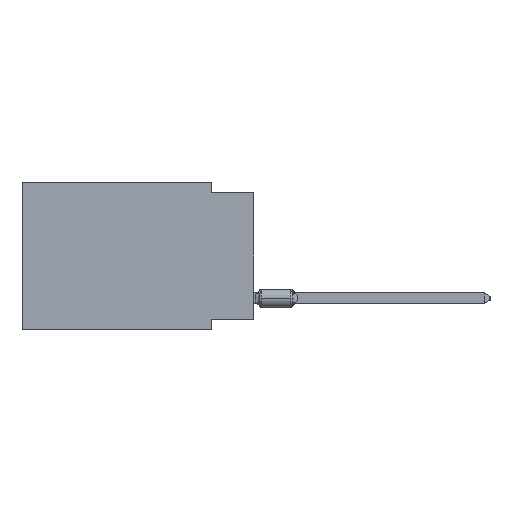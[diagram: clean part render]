
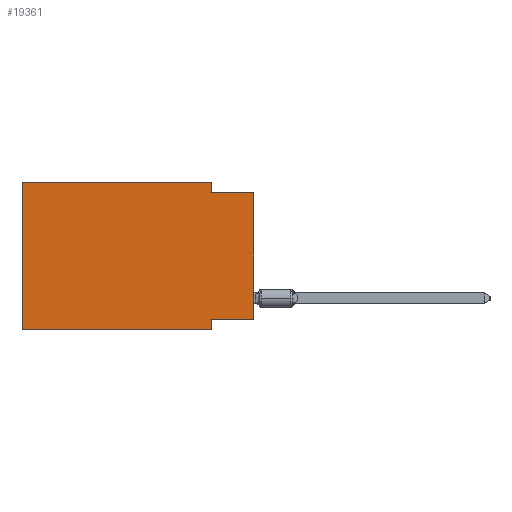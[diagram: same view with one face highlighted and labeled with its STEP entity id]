
A CAD part, left-side view. The second image highlights one B-rep face of the part: STEP entity #19361.
In plain terms, the highlighted planar face has unit normal (-1, 0, 0).
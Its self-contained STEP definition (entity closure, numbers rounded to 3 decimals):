
#1639 = ORIENTED_EDGE ( 'NONE', *, *, #43467, .F. ) ;
#3488 = DIRECTION ( 'NONE',  ( 0., 0., 1. ) ) ;
#3862 = ORIENTED_EDGE ( 'NONE', *, *, #51844, .T. ) ;
#6114 = DIRECTION ( 'NONE',  ( 0., -1., 0. ) ) ;
#6703 = EDGE_CURVE ( 'NONE', #42554, #51807, #19108, .T. ) ;
#8383 = EDGE_CURVE ( 'NONE', #15326, #42554, #37572, .T. ) ;
#8854 = AXIS2_PLACEMENT_3D ( 'NONE', #10410, #52341, #43872 ) ;
#9474 = EDGE_LOOP ( 'NONE', ( #3862, #1639, #18392, #10785, #9512, #40778, #19941, #19553 ) ) ;
#9512 = ORIENTED_EDGE ( 'NONE', *, *, #19896, .F. ) ;
#10410 = CARTESIAN_POINT ( 'NONE',  ( 0., 13.97, 0. ) ) ;
#10785 = ORIENTED_EDGE ( 'NONE', *, *, #8383, .F. ) ;
#12265 = VERTEX_POINT ( 'NONE', #48826 ) ;
#13125 = VERTEX_POINT ( 'NONE', #30211 ) ;
#13335 = CARTESIAN_POINT ( 'NONE',  ( 0., 2.54, -8.255 ) ) ;
#13735 = LINE ( 'NONE', #21696, #19118 ) ;
#15326 = VERTEX_POINT ( 'NONE', #28820 ) ;
#15983 = CARTESIAN_POINT ( 'NONE',  ( 0., 2.54, 0. ) ) ;
#18392 = ORIENTED_EDGE ( 'NONE', *, *, #6703, .F. ) ;
#19108 = LINE ( 'NONE', #24293, #47447 ) ;
#19118 = VECTOR ( 'NONE', #42534, 1000. ) ;
#19361 = ADVANCED_FACE ( 'NONE', ( #30689 ), #47964, .F. ) ;
#19553 = ORIENTED_EDGE ( 'NONE', *, *, #29932, .F. ) ;
#19896 = EDGE_CURVE ( 'NONE', #23917, #15326, #32258, .T. ) ;
#19941 = ORIENTED_EDGE ( 'NONE', *, *, #35292, .F. ) ;
#21696 = CARTESIAN_POINT ( 'NONE',  ( 0., 0., 0. ) ) ;
#23917 = VERTEX_POINT ( 'NONE', #50975 ) ;
#24293 = CARTESIAN_POINT ( 'NONE',  ( 0., 2.54, 0. ) ) ;
#27291 = LINE ( 'NONE', #35233, #31234 ) ;
#28150 = VECTOR ( 'NONE', #3488, 1000. ) ;
#28518 = CARTESIAN_POINT ( 'NONE',  ( 0., 13.97, 0. ) ) ;
#28728 = VERTEX_POINT ( 'NONE', #31023 ) ;
#28820 = CARTESIAN_POINT ( 'NONE',  ( 0., 13.97, 0. ) ) ;
#29932 = EDGE_CURVE ( 'NONE', #28728, #45752, #45809, .T. ) ;
#30072 = VECTOR ( 'NONE', #49626, 1000. ) ;
#30211 = CARTESIAN_POINT ( 'NONE',  ( 0., 2.54, -8.89 ) ) ;
#30689 = FACE_OUTER_BOUND ( 'NONE', #9474, .T. ) ;
#31023 = CARTESIAN_POINT ( 'NONE',  ( 0., 0., -8.255 ) ) ;
#31234 = VECTOR ( 'NONE', #51956, 1000. ) ;
#32258 = LINE ( 'NONE', #48981, #28150 ) ;
#32354 = CARTESIAN_POINT ( 'NONE',  ( 0., 0., -8.255 ) ) ;
#33465 = DIRECTION ( 'NONE',  ( 0., 1., 0. ) ) ;
#35233 = CARTESIAN_POINT ( 'NONE',  ( 0., 13.97, -8.89 ) ) ;
#35292 = EDGE_CURVE ( 'NONE', #45752, #13125, #35923, .T. ) ;
#35443 = CARTESIAN_POINT ( 'NONE',  ( 0., 0., -0.635 ) ) ;
#35923 = LINE ( 'NONE', #36194, #36417 ) ;
#36035 = EDGE_CURVE ( 'NONE', #23917, #13125, #27291, .T. ) ;
#36194 = CARTESIAN_POINT ( 'NONE',  ( 0., 2.54, -8.89 ) ) ;
#36417 = VECTOR ( 'NONE', #52635, 1000. ) ;
#37572 = LINE ( 'NONE', #28518, #30072 ) ;
#37889 = CARTESIAN_POINT ( 'NONE',  ( 0., 2.54, -0.635 ) ) ;
#38837 = VECTOR ( 'NONE', #33465, 1000. ) ;
#39285 = LINE ( 'NONE', #35443, #46758 ) ;
#40778 = ORIENTED_EDGE ( 'NONE', *, *, #36035, .T. ) ;
#42534 = DIRECTION ( 'NONE',  ( 0., 0., 1. ) ) ;
#42554 = VERTEX_POINT ( 'NONE', #15983 ) ;
#43467 = EDGE_CURVE ( 'NONE', #51807, #12265, #39285, .T. ) ;
#43872 = DIRECTION ( 'NONE',  ( 0., 0., -1. ) ) ;
#45752 = VERTEX_POINT ( 'NONE', #13335 ) ;
#45809 = LINE ( 'NONE', #32354, #38837 ) ;
#46758 = VECTOR ( 'NONE', #6114, 1000. ) ;
#47447 = VECTOR ( 'NONE', #48413, 1000. ) ;
#47964 = PLANE ( 'NONE',  #8854 ) ;
#48413 = DIRECTION ( 'NONE',  ( 0., 0., -1. ) ) ;
#48826 = CARTESIAN_POINT ( 'NONE',  ( 0., 0., -0.635 ) ) ;
#48981 = CARTESIAN_POINT ( 'NONE',  ( 0., 13.97, 0. ) ) ;
#49626 = DIRECTION ( 'NONE',  ( 0., -1., 0. ) ) ;
#50975 = CARTESIAN_POINT ( 'NONE',  ( 0., 13.97, -8.89 ) ) ;
#51807 = VERTEX_POINT ( 'NONE', #37889 ) ;
#51844 = EDGE_CURVE ( 'NONE', #28728, #12265, #13735, .T. ) ;
#51956 = DIRECTION ( 'NONE',  ( 0., -1., 0. ) ) ;
#52341 = DIRECTION ( 'NONE',  ( 1., 0., 0. ) ) ;
#52635 = DIRECTION ( 'NONE',  ( 0., 0., -1. ) ) ;
